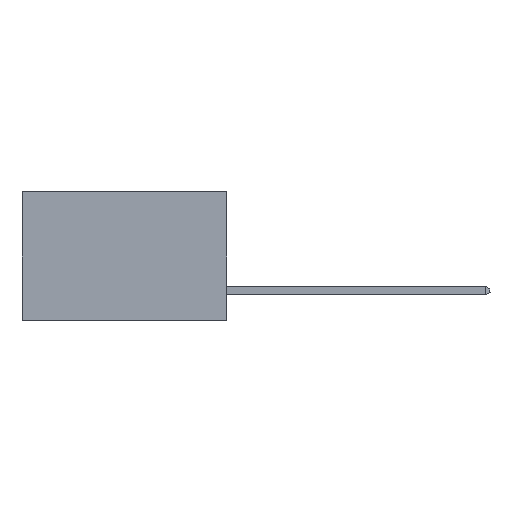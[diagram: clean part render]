
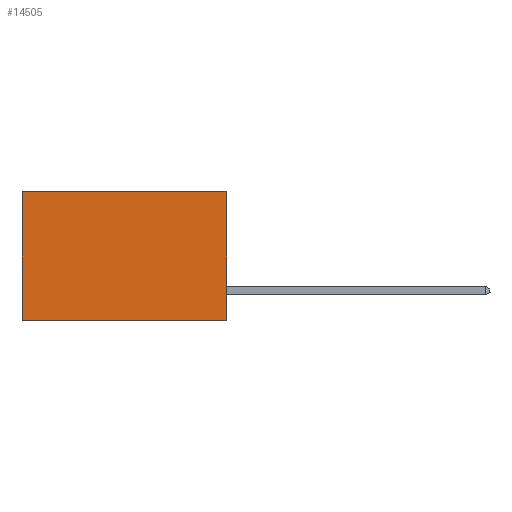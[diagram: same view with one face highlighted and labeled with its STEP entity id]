
A CAD part, left-side view. The second image highlights one B-rep face of the part: STEP entity #14505.
In plain terms, the highlighted planar face has unit normal (-1, 0, 0).
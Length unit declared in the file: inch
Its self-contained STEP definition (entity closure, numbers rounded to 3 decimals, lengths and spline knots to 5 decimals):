
#30 = FACE_OUTER_BOUND ( 'NONE', #1113, .T. ) ;
#1113 = EDGE_LOOP ( 'NONE', ( #22845, #7469, #3268, #13847 ) ) ;
#1626 = LINE ( 'NONE', #6932, #10874 ) ;
#1993 = VERTEX_POINT ( 'NONE', #9553 ) ;
#3268 = ORIENTED_EDGE ( 'NONE', *, *, #12182, .F. ) ;
#3621 = LINE ( 'NONE', #18012, #23295 ) ;
#3972 = LINE ( 'NONE', #21937, #14221 ) ;
#4030 = DIRECTION ( 'NONE',  ( 0., 0., -1. ) ) ;
#6419 = DIRECTION ( 'NONE',  ( 0., 1., 0. ) ) ;
#6932 = CARTESIAN_POINT ( 'NONE',  ( 0.277, 0., -0.37 ) ) ;
#7126 = EDGE_CURVE ( 'NONE', #12271, #16932, #1626, .T. ) ;
#7362 = LINE ( 'NONE', #11764, #16244 ) ;
#7469 = ORIENTED_EDGE ( 'NONE', *, *, #7126, .F. ) ;
#8996 = PLANE ( 'NONE',  #22323 ) ;
#9435 = CARTESIAN_POINT ( 'NONE',  ( 0.277, 0.59, -0.37 ) ) ;
#9553 = CARTESIAN_POINT ( 'NONE',  ( 0.277, 0.59, 0. ) ) ;
#10874 = VECTOR ( 'NONE', #6419, 39.37008 ) ;
#11146 = DIRECTION ( 'NONE',  ( 1., 0., 0. ) ) ;
#11535 = EDGE_CURVE ( 'NONE', #21605, #1993, #3972, .T. ) ;
#11764 = CARTESIAN_POINT ( 'NONE',  ( 0.277, 0.59, -0.37 ) ) ;
#12182 = EDGE_CURVE ( 'NONE', #21605, #12271, #3621, .T. ) ;
#12271 = VERTEX_POINT ( 'NONE', #16256 ) ;
#13847 = ORIENTED_EDGE ( 'NONE', *, *, #11535, .T. ) ;
#14221 = VECTOR ( 'NONE', #18524, 39.37008 ) ;
#14505 = ADVANCED_FACE ( 'NONE', ( #30 ), #8996, .F. ) ;
#15718 = CARTESIAN_POINT ( 'NONE',  ( 0.277, 0., 0. ) ) ;
#16244 = VECTOR ( 'NONE', #4030, 39.37008 ) ;
#16256 = CARTESIAN_POINT ( 'NONE',  ( 0.277, 0., -0.37 ) ) ;
#16932 = VERTEX_POINT ( 'NONE', #9435 ) ;
#17638 = DIRECTION ( 'NONE',  ( 0., 0., -1. ) ) ;
#18012 = CARTESIAN_POINT ( 'NONE',  ( 0.277, 0., -0.37 ) ) ;
#18524 = DIRECTION ( 'NONE',  ( 0., 1., 0. ) ) ;
#19506 = EDGE_CURVE ( 'NONE', #1993, #16932, #7362, .T. ) ;
#20535 = CARTESIAN_POINT ( 'NONE',  ( 0.277, 0., -0.37 ) ) ;
#21605 = VERTEX_POINT ( 'NONE', #15718 ) ;
#21937 = CARTESIAN_POINT ( 'NONE',  ( 0.277, 0., 0. ) ) ;
#22323 = AXIS2_PLACEMENT_3D ( 'NONE', #20535, #11146, #24237 ) ;
#22845 = ORIENTED_EDGE ( 'NONE', *, *, #19506, .T. ) ;
#23295 = VECTOR ( 'NONE', #17638, 39.37008 ) ;
#24237 = DIRECTION ( 'NONE',  ( 0., 0., -1. ) ) ;
